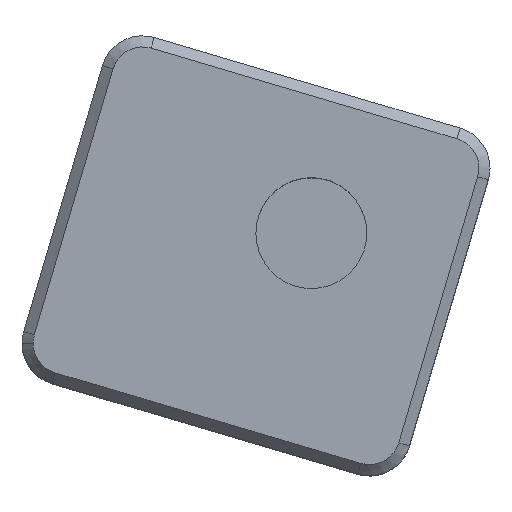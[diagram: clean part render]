
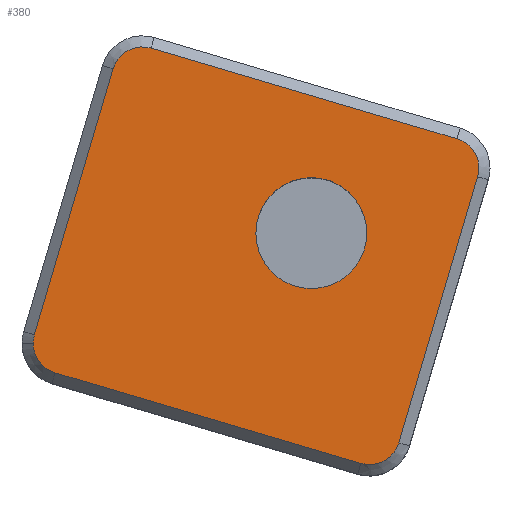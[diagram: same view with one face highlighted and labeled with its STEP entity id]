
A CAD part, top view. The second image highlights one B-rep face of the part: STEP entity #380.
In plain terms, the highlighted planar face has unit normal (0, 0, 1).
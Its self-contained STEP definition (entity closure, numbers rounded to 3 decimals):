
#27 = ORIENTED_EDGE ( 'NONE', *, *, #293, .T. ) ;
#43 = DIRECTION ( 'NONE',  ( -0.959, 0.284, 0. ) ) ;
#44 = VERTEX_POINT ( 'NONE', #704 ) ;
#56 = VERTEX_POINT ( 'NONE', #867 ) ;
#65 = EDGE_CURVE ( 'NONE', #1037, #128, #1136, .T. ) ;
#70 = EDGE_CURVE ( 'NONE', #540, #571, #426, .T. ) ;
#87 = EDGE_CURVE ( 'NONE', #1106, #44, #281, .T. ) ;
#109 = DIRECTION ( 'NONE',  ( -0.284, -0.959, 0. ) ) ;
#121 = ORIENTED_EDGE ( 'NONE', *, *, #481, .T. ) ;
#128 = VERTEX_POINT ( 'NONE', #624 ) ;
#135 = CARTESIAN_POINT ( 'NONE',  ( -32.142, -25.562, -15. ) ) ;
#157 = CARTESIAN_POINT ( 'NONE',  ( -20.06, -29.141, -15. ) ) ;
#158 = ORIENTED_EDGE ( 'NONE', *, *, #897, .T. ) ;
#162 = DIRECTION ( 'NONE',  ( 0., 0., -1. ) ) ;
#165 = AXIS2_PLACEMENT_3D ( 'NONE', #135, #506, #671 ) ;
#184 = FACE_OUTER_BOUND ( 'NONE', #1034, .T. ) ;
#223 = VECTOR ( 'NONE', #377, 1000. ) ;
#273 = EDGE_CURVE ( 'NONE', #741, #540, #445, .T. ) ;
#279 = CARTESIAN_POINT ( 'NONE',  ( -17.22, -19.553, -15. ) ) ;
#281 = CIRCLE ( 'NONE', #791, 1.1 ) ;
#293 = EDGE_CURVE ( 'NONE', #584, #1106, #739, .T. ) ;
#319 = CARTESIAN_POINT ( 'NONE',  ( -29.301, -15.974, -15. ) ) ;
#347 = DIRECTION ( 'NONE',  ( 0., 0., 1. ) ) ;
#357 = PLANE ( 'NONE',  #657 ) ;
#377 = DIRECTION ( 'NONE',  ( 0.284, 0.959, 0. ) ) ;
#380 = ADVANCED_FACE ( 'NONE', ( #824, #184 ), #357, .T. ) ;
#400 = EDGE_LOOP ( 'NONE', ( #672, #1099 ) ) ;
#411 = VERTEX_POINT ( 'NONE', #459 ) ;
#426 = CIRCLE ( 'NONE', #1021, 1.1 ) ;
#429 = CIRCLE ( 'NONE', #955, 1.1 ) ;
#435 = CARTESIAN_POINT ( 'NONE',  ( -23.215, -23.585, -15. ) ) ;
#445 = LINE ( 'NONE', #807, #615 ) ;
#459 = CARTESIAN_POINT ( 'NONE',  ( -17.963, -18.186, -15. ) ) ;
#481 = EDGE_CURVE ( 'NONE', #411, #56, #493, .T. ) ;
#493 = LINE ( 'NONE', #860, #504 ) ;
#504 = VECTOR ( 'NONE', #43, 1000. ) ;
#506 = DIRECTION ( 'NONE',  ( 0., 0., 1. ) ) ;
#513 = CARTESIAN_POINT ( 'NONE',  ( -21.428, -29.883, -15. ) ) ;
#526 = DIRECTION ( 'NONE',  ( -1., 0., 0. ) ) ;
#538 = DIRECTION ( 'NONE',  ( 0., 1., 0. ) ) ;
#540 = VERTEX_POINT ( 'NONE', #513 ) ;
#543 = CARTESIAN_POINT ( 'NONE',  ( -23.215, -21.585, -15. ) ) ;
#550 = CARTESIAN_POINT ( 'NONE',  ( -32.142, -25.562, -15. ) ) ;
#554 = CARTESIAN_POINT ( 'NONE',  ( -30.356, -15.662, -15. ) ) ;
#555 = EDGE_CURVE ( 'NONE', #56, #584, #429, .T. ) ;
#571 = VERTEX_POINT ( 'NONE', #157 ) ;
#573 = LINE ( 'NONE', #1093, #223 ) ;
#584 = VERTEX_POINT ( 'NONE', #1061 ) ;
#609 = ORIENTED_EDGE ( 'NONE', *, *, #698, .T. ) ;
#615 = VECTOR ( 'NONE', #757, 1000. ) ;
#622 = EDGE_CURVE ( 'NONE', #128, #1037, #736, .T. ) ;
#624 = CARTESIAN_POINT ( 'NONE',  ( -23.215, -19.585, -15. ) ) ;
#644 = CARTESIAN_POINT ( 'NONE',  ( -33.196, -25.25, -15. ) ) ;
#657 = AXIS2_PLACEMENT_3D ( 'NONE', #1030, #719, #1076 ) ;
#668 = ORIENTED_EDGE ( 'NONE', *, *, #555, .T. ) ;
#671 = DIRECTION ( 'NONE',  ( -1., 0., 0. ) ) ;
#672 = ORIENTED_EDGE ( 'NONE', *, *, #65, .T. ) ;
#678 = ORIENTED_EDGE ( 'NONE', *, *, #1123, .T. ) ;
#690 = CARTESIAN_POINT ( 'NONE',  ( -21.115, -28.829, -15. ) ) ;
#698 = EDGE_CURVE ( 'NONE', #823, #411, #1053, .T. ) ;
#704 = CARTESIAN_POINT ( 'NONE',  ( -33.242, -25.562, -15. ) ) ;
#705 = DIRECTION ( 'NONE',  ( 0., 0., 1. ) ) ;
#709 = DIRECTION ( 'NONE',  ( 0., 0., 1. ) ) ;
#719 = DIRECTION ( 'NONE',  ( 0., 0., 1. ) ) ;
#734 = AXIS2_PLACEMENT_3D ( 'NONE', #543, #162, #1083 ) ;
#736 = CIRCLE ( 'NONE', #734, 2. ) ;
#739 = LINE ( 'NONE', #554, #1156 ) ;
#741 = VERTEX_POINT ( 'NONE', #755 ) ;
#752 = CIRCLE ( 'NONE', #165, 1.1 ) ;
#755 = CARTESIAN_POINT ( 'NONE',  ( -32.454, -26.617, -15. ) ) ;
#757 = DIRECTION ( 'NONE',  ( 0.959, -0.284, 0. ) ) ;
#768 = ORIENTED_EDGE ( 'NONE', *, *, #87, .T. ) ;
#791 = AXIS2_PLACEMENT_3D ( 'NONE', #550, #1163, #908 ) ;
#797 = CARTESIAN_POINT ( 'NONE',  ( -23.215, -21.585, -15. ) ) ;
#807 = CARTESIAN_POINT ( 'NONE',  ( -32.454, -26.617, -15. ) ) ;
#823 = VERTEX_POINT ( 'NONE', #279 ) ;
#824 = FACE_BOUND ( 'NONE', #400, .T. ) ;
#838 = ORIENTED_EDGE ( 'NONE', *, *, #273, .T. ) ;
#859 = DIRECTION ( 'NONE',  ( -1., 0., 0. ) ) ;
#860 = CARTESIAN_POINT ( 'NONE',  ( -17.963, -18.186, -15. ) ) ;
#867 = CARTESIAN_POINT ( 'NONE',  ( -28.989, -14.92, -15. ) ) ;
#897 = EDGE_CURVE ( 'NONE', #44, #741, #752, .T. ) ;
#899 = AXIS2_PLACEMENT_3D ( 'NONE', #797, #1130, #1148 ) ;
#908 = DIRECTION ( 'NONE',  ( -1., 0., 0. ) ) ;
#955 = AXIS2_PLACEMENT_3D ( 'NONE', #319, #705, #526 ) ;
#1021 = AXIS2_PLACEMENT_3D ( 'NONE', #690, #347, #859 ) ;
#1030 = CARTESIAN_POINT ( 'NONE',  ( -25.191, -23.278, -15. ) ) ;
#1033 = AXIS2_PLACEMENT_3D ( 'NONE', #1154, #709, #538 ) ;
#1034 = EDGE_LOOP ( 'NONE', ( #1058, #678, #609, #121, #668, #27, #768, #158, #838 ) ) ;
#1037 = VERTEX_POINT ( 'NONE', #435 ) ;
#1053 = CIRCLE ( 'NONE', #1033, 1.1 ) ;
#1058 = ORIENTED_EDGE ( 'NONE', *, *, #70, .T. ) ;
#1061 = CARTESIAN_POINT ( 'NONE',  ( -30.356, -15.662, -15. ) ) ;
#1076 = DIRECTION ( 'NONE',  ( 0., -1., 0. ) ) ;
#1083 = DIRECTION ( 'NONE',  ( 0., -1., 0. ) ) ;
#1093 = CARTESIAN_POINT ( 'NONE',  ( -20.06, -29.141, -15. ) ) ;
#1099 = ORIENTED_EDGE ( 'NONE', *, *, #622, .T. ) ;
#1106 = VERTEX_POINT ( 'NONE', #644 ) ;
#1123 = EDGE_CURVE ( 'NONE', #571, #823, #573, .T. ) ;
#1130 = DIRECTION ( 'NONE',  ( 0., 0., -1. ) ) ;
#1136 = CIRCLE ( 'NONE', #899, 2. ) ;
#1148 = DIRECTION ( 'NONE',  ( 0., -1., 0. ) ) ;
#1154 = CARTESIAN_POINT ( 'NONE',  ( -18.275, -19.24, -15. ) ) ;
#1156 = VECTOR ( 'NONE', #109, 1000. ) ;
#1163 = DIRECTION ( 'NONE',  ( 0., 0., 1. ) ) ;
